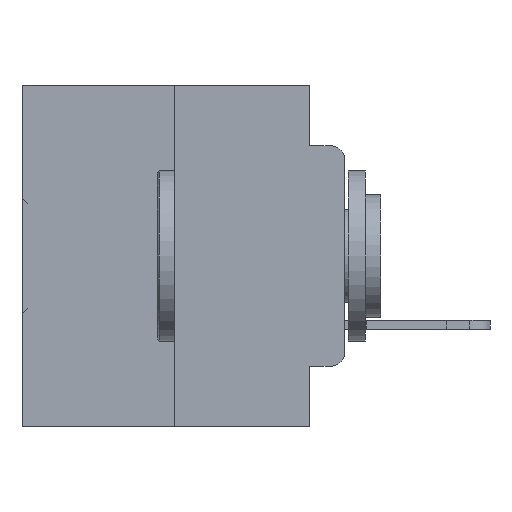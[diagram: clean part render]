
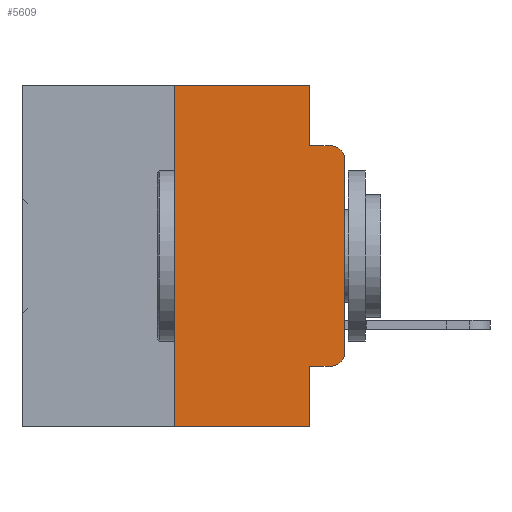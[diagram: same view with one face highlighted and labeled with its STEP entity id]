
A CAD part, left-side view. The second image highlights one B-rep face of the part: STEP entity #5609.
In plain terms, the highlighted planar face has unit normal (-1, 0, 0).
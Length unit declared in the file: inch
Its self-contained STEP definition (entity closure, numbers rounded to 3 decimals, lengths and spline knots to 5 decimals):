
#431 = VERTEX_POINT ( 'NONE', #6814 ) ;
#878 = EDGE_CURVE ( 'NONE', #431, #10997, #6089, .T. ) ;
#1154 = ORIENTED_EDGE ( 'NONE', *, *, #20151, .T. ) ;
#1823 = CARTESIAN_POINT ( 'NONE',  ( 0., 0.02, -0.4115 ) ) ;
#1921 = CARTESIAN_POINT ( 'NONE',  ( 0., 0.25, 0. ) ) ;
#2792 = EDGE_CURVE ( 'NONE', #431, #35724, #19899, .T. ) ;
#2850 = EDGE_CURVE ( 'NONE', #5416, #11947, #32760, .T. ) ;
#3054 = ORIENTED_EDGE ( 'NONE', *, *, #878, .T. ) ;
#3471 = VECTOR ( 'NONE', #18353, 39.37008 ) ;
#3926 = EDGE_LOOP ( 'NONE', ( #35791, #1154, #11433, #15949, #7951, #27467, #16022, #30481, #3054, #35095 ) ) ;
#4701 = EDGE_CURVE ( 'NONE', #36079, #5416, #21969, .T. ) ;
#4797 = VERTEX_POINT ( 'NONE', #26807 ) ;
#5283 = CARTESIAN_POINT ( 'NONE',  ( 0., 0.25, -0.5 ) ) ;
#5416 = VERTEX_POINT ( 'NONE', #1921 ) ;
#5434 = VECTOR ( 'NONE', #29741, 39.37008 ) ;
#5608 = CIRCLE ( 'NONE', #31400, 0.02 ) ;
#5609 = ADVANCED_FACE ( 'NONE', ( #27492 ), #18775, .F. ) ;
#5977 = CARTESIAN_POINT ( 'NONE',  ( 0., 0.051, -0.4115 ) ) ;
#6075 = AXIS2_PLACEMENT_3D ( 'NONE', #13967, #15539, #9248 ) ;
#6089 = LINE ( 'NONE', #5977, #14590 ) ;
#6229 = DIRECTION ( 'NONE',  ( -1., 0., 0. ) ) ;
#6634 = EDGE_CURVE ( 'NONE', #11947, #11813, #11068, .T. ) ;
#6652 = DIRECTION ( 'NONE',  ( 0., -1., 0. ) ) ;
#6814 = CARTESIAN_POINT ( 'NONE',  ( 0., 0.051, -0.4115 ) ) ;
#7844 = LINE ( 'NONE', #33966, #14506 ) ;
#7951 = ORIENTED_EDGE ( 'NONE', *, *, #2850, .F. ) ;
#8939 = CARTESIAN_POINT ( 'NONE',  ( 0., 0.051, -0.0885 ) ) ;
#9109 = CARTESIAN_POINT ( 'NONE',  ( 0., 0.051, -0.5 ) ) ;
#9248 = DIRECTION ( 'NONE',  ( 0., 0., -1. ) ) ;
#9565 = CARTESIAN_POINT ( 'NONE',  ( 0., 0.051, -0.0885 ) ) ;
#9572 = EDGE_CURVE ( 'NONE', #36079, #35724, #13078, .T. ) ;
#10559 = CARTESIAN_POINT ( 'NONE',  ( 0., 0.473, 0. ) ) ;
#10997 = VERTEX_POINT ( 'NONE', #1823 ) ;
#11068 = LINE ( 'NONE', #18958, #3471 ) ;
#11433 = ORIENTED_EDGE ( 'NONE', *, *, #18233, .F. ) ;
#11813 = VERTEX_POINT ( 'NONE', #8939 ) ;
#11947 = VERTEX_POINT ( 'NONE', #29177 ) ;
#12382 = CARTESIAN_POINT ( 'NONE',  ( 0., 0.02, -0.1085 ) ) ;
#13078 = LINE ( 'NONE', #30134, #5434 ) ;
#13117 = VECTOR ( 'NONE', #16247, 39.37008 ) ;
#13967 = CARTESIAN_POINT ( 'NONE',  ( 0., 0.473, 0. ) ) ;
#14450 = DIRECTION ( 'NONE',  ( 0., 0., 1. ) ) ;
#14506 = VECTOR ( 'NONE', #14450, 39.37008 ) ;
#14590 = VECTOR ( 'NONE', #32824, 39.37008 ) ;
#14764 = CARTESIAN_POINT ( 'NONE',  ( 0., 0., -0.3915 ) ) ;
#14896 = LINE ( 'NONE', #9565, #21701 ) ;
#15234 = DIRECTION ( 'NONE',  ( 0., 0., -1. ) ) ;
#15539 = DIRECTION ( 'NONE',  ( 1., 0., 0. ) ) ;
#15949 = ORIENTED_EDGE ( 'NONE', *, *, #6634, .F. ) ;
#16022 = ORIENTED_EDGE ( 'NONE', *, *, #9572, .T. ) ;
#16247 = DIRECTION ( 'NONE',  ( 0., 0., -1. ) ) ;
#17882 = DIRECTION ( 'NONE',  ( 0., 0., 1. ) ) ;
#18105 = VERTEX_POINT ( 'NONE', #14764 ) ;
#18140 = CARTESIAN_POINT ( 'NONE',  ( 0., 0.25, 0. ) ) ;
#18233 = EDGE_CURVE ( 'NONE', #11813, #4797, #14896, .T. ) ;
#18353 = DIRECTION ( 'NONE',  ( 0., 0., -1. ) ) ;
#18775 = PLANE ( 'NONE',  #6075 ) ;
#18958 = CARTESIAN_POINT ( 'NONE',  ( 0., 0.051, 0. ) ) ;
#19899 = LINE ( 'NONE', #29653, #13117 ) ;
#20151 = EDGE_CURVE ( 'NONE', #21540, #4797, #25792, .T. ) ;
#21540 = VERTEX_POINT ( 'NONE', #26560 ) ;
#21701 = VECTOR ( 'NONE', #6652, 39.37008 ) ;
#21851 = AXIS2_PLACEMENT_3D ( 'NONE', #12382, #31971, #15234 ) ;
#21969 = LINE ( 'NONE', #18140, #30122 ) ;
#22035 = EDGE_CURVE ( 'NONE', #18105, #21540, #7844, .T. ) ;
#23397 = CARTESIAN_POINT ( 'NONE',  ( 0., 0.02, -0.3915 ) ) ;
#25792 = CIRCLE ( 'NONE', #21851, 0.02 ) ;
#26140 = DIRECTION ( 'NONE',  ( 0., 0., -1. ) ) ;
#26414 = EDGE_CURVE ( 'NONE', #10997, #18105, #5608, .T. ) ;
#26560 = CARTESIAN_POINT ( 'NONE',  ( 0., 0., -0.1085 ) ) ;
#26807 = CARTESIAN_POINT ( 'NONE',  ( 0., 0.02, -0.0885 ) ) ;
#27467 = ORIENTED_EDGE ( 'NONE', *, *, #4701, .F. ) ;
#27492 = FACE_OUTER_BOUND ( 'NONE', #3926, .T. ) ;
#29177 = CARTESIAN_POINT ( 'NONE',  ( 0., 0.051, 0. ) ) ;
#29577 = DIRECTION ( 'NONE',  ( 0., -1., 0. ) ) ;
#29653 = CARTESIAN_POINT ( 'NONE',  ( 0., 0.051, 0. ) ) ;
#29741 = DIRECTION ( 'NONE',  ( 0., -1., 0. ) ) ;
#30122 = VECTOR ( 'NONE', #17882, 39.37008 ) ;
#30134 = CARTESIAN_POINT ( 'NONE',  ( 0., 0.473, -0.5 ) ) ;
#30481 = ORIENTED_EDGE ( 'NONE', *, *, #2792, .F. ) ;
#31400 = AXIS2_PLACEMENT_3D ( 'NONE', #23397, #6229, #26140 ) ;
#31945 = VECTOR ( 'NONE', #29577, 39.37008 ) ;
#31971 = DIRECTION ( 'NONE',  ( -1., 0., 0. ) ) ;
#32760 = LINE ( 'NONE', #10559, #31945 ) ;
#32824 = DIRECTION ( 'NONE',  ( 0., -1., 0. ) ) ;
#33966 = CARTESIAN_POINT ( 'NONE',  ( 0., 0., 0. ) ) ;
#35095 = ORIENTED_EDGE ( 'NONE', *, *, #26414, .T. ) ;
#35724 = VERTEX_POINT ( 'NONE', #9109 ) ;
#35791 = ORIENTED_EDGE ( 'NONE', *, *, #22035, .T. ) ;
#36079 = VERTEX_POINT ( 'NONE', #5283 ) ;
